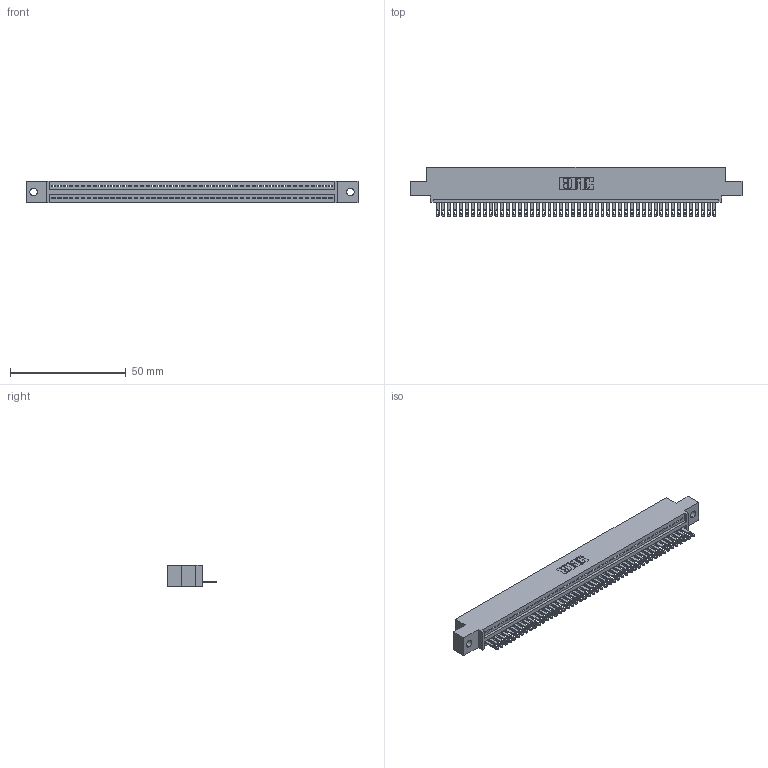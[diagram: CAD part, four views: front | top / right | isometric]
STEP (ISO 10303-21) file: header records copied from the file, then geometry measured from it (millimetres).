
FILE_DESCRIPTION (( 'STEP AP203' ), '1' );
FILE_NAME ('345-048-500-402.STEP', '2018-09-11T08:47:30', ( '' ), ( '' ), 'SwSTEP 2.0', 'SolidWorks 2016', '' );
FILE_SCHEMA (( 'CONFIG_CONTROL_DESIGN' ));
Length unit declared in the file: inch
Products named in the file (3): 345 Part_0.110 Offset - 0.128 Dia; 345-292-001_345-293-100; 345-048-500-402
Assembly tree (49 placements, depth 2):
  345-048-500-402
    345 Part_0.110 Offset - 0.128 Dia
    345-292-001_345-293-100  x48
Bounding box: 143.13 x 21.51 x 9.4 mm (x, y, z)
Volume: 13563.3 mm3; surface area: 18024.2 mm2
Topology: 49 solids, 49 shells, 2722 faces, 8417 edges, 5610 vertices
Faces by surface type: plane 1716, cylinder 1006
Entity records: 35383 total; most frequent: CARTESIAN_POINT 6136, ORIENTED_EDGE 6118, DIRECTION 5351, EDGE_CURVE 3059, LINE 2731, VECTOR 2731, VERTEX_POINT 2038, AXIS2_PLACEMENT_3D 1310
